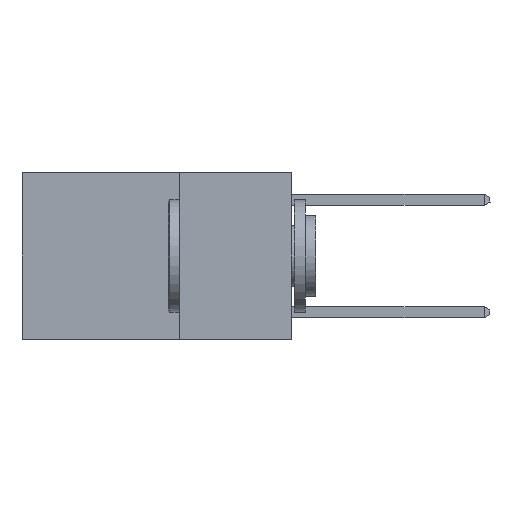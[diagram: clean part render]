
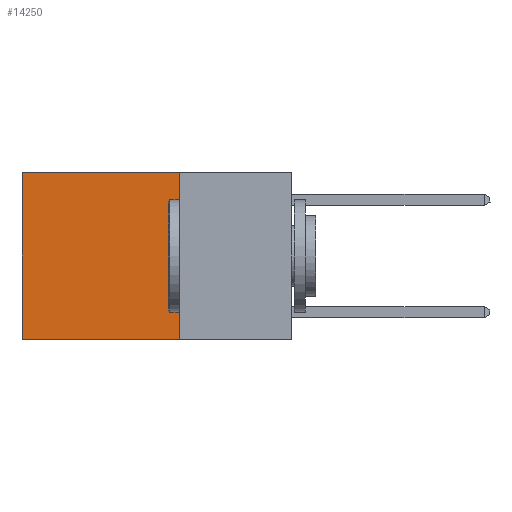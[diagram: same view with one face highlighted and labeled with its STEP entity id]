
A CAD part, left-side view. The second image highlights one B-rep face of the part: STEP entity #14250.
In plain terms, the highlighted planar face has unit normal (-1, 0, 0).
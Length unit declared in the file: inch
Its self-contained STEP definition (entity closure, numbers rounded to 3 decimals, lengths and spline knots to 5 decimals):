
#155 = EDGE_CURVE ( 'NONE', #2223, #4427, #16339, .T. ) ;
#577 = VECTOR ( 'NONE', #943, 39.37008 ) ;
#756 = CARTESIAN_POINT ( 'NONE',  ( 0.2625, 0.6, 0. ) ) ;
#943 = DIRECTION ( 'NONE',  ( 0., 1., 0. ) ) ;
#2123 = ORIENTED_EDGE ( 'NONE', *, *, #6828, .T. ) ;
#2223 = VERTEX_POINT ( 'NONE', #756 ) ;
#2811 = VECTOR ( 'NONE', #3816, 39.37008 ) ;
#3080 = CARTESIAN_POINT ( 'NONE',  ( 0.2625, 0.25, 0. ) ) ;
#3662 = AXIS2_PLACEMENT_3D ( 'NONE', #7317, #11241, #8827 ) ;
#3816 = DIRECTION ( 'NONE',  ( 0., 1., 0. ) ) ;
#4427 = VERTEX_POINT ( 'NONE', #8513 ) ;
#5787 = PLANE ( 'NONE',  #3662 ) ;
#6061 = FACE_OUTER_BOUND ( 'NONE', #16456, .T. ) ;
#6828 = EDGE_CURVE ( 'NONE', #15882, #2223, #16200, .T. ) ;
#7317 = CARTESIAN_POINT ( 'NONE',  ( 0.2625, 0.25, 0. ) ) ;
#7836 = EDGE_CURVE ( 'NONE', #15882, #8176, #16746, .T. ) ;
#8176 = VERTEX_POINT ( 'NONE', #13255 ) ;
#8196 = CARTESIAN_POINT ( 'NONE',  ( 0.2625, 0.6, 0. ) ) ;
#8513 = CARTESIAN_POINT ( 'NONE',  ( 0.2625, 0.6, -0.37 ) ) ;
#8827 = DIRECTION ( 'NONE',  ( 0., 0., -1. ) ) ;
#8878 = ORIENTED_EDGE ( 'NONE', *, *, #7836, .F. ) ;
#9402 = CARTESIAN_POINT ( 'NONE',  ( 0.2625, 0.25, 0. ) ) ;
#10127 = ORIENTED_EDGE ( 'NONE', *, *, #155, .T. ) ;
#11110 = DIRECTION ( 'NONE',  ( 0., 0., -1. ) ) ;
#11241 = DIRECTION ( 'NONE',  ( 1., 0., 0. ) ) ;
#11468 = VECTOR ( 'NONE', #11110, 39.37008 ) ;
#12249 = VECTOR ( 'NONE', #14815, 39.37008 ) ;
#13187 = LINE ( 'NONE', #14533, #2811 ) ;
#13255 = CARTESIAN_POINT ( 'NONE',  ( 0.2625, 0.25, -0.37 ) ) ;
#14250 = ADVANCED_FACE ( 'NONE', ( #6061 ), #5787, .F. ) ;
#14533 = CARTESIAN_POINT ( 'NONE',  ( 0.2625, 0.25, -0.37 ) ) ;
#14815 = DIRECTION ( 'NONE',  ( 0., 0., -1. ) ) ;
#14931 = EDGE_CURVE ( 'NONE', #8176, #4427, #13187, .T. ) ;
#15882 = VERTEX_POINT ( 'NONE', #17181 ) ;
#16200 = LINE ( 'NONE', #9402, #577 ) ;
#16339 = LINE ( 'NONE', #8196, #12249 ) ;
#16456 = EDGE_LOOP ( 'NONE', ( #10127, #16556, #8878, #2123 ) ) ;
#16556 = ORIENTED_EDGE ( 'NONE', *, *, #14931, .F. ) ;
#16746 = LINE ( 'NONE', #3080, #11468 ) ;
#17181 = CARTESIAN_POINT ( 'NONE',  ( 0.2625, 0.25, 0. ) ) ;
